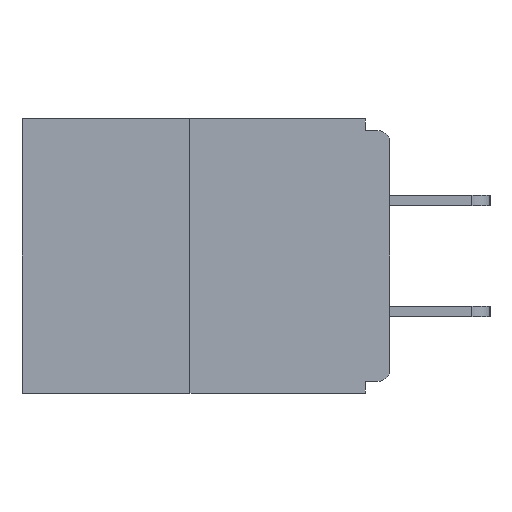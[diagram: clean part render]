
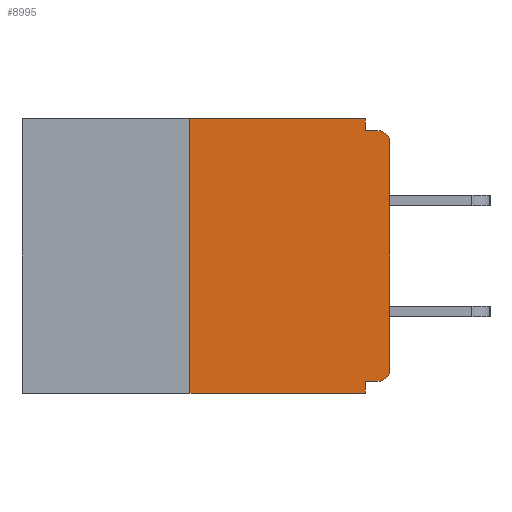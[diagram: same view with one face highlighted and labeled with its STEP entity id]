
A CAD part, left-side view. The second image highlights one B-rep face of the part: STEP entity #8995.
In plain terms, the highlighted planar face has unit normal (-1, 0, 0).
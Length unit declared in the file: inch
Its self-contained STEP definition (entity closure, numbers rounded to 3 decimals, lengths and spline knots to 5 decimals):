
#594 = VECTOR ( 'NONE', #9159, 39.37008 ) ;
#635 = CARTESIAN_POINT ( 'NONE',  ( 0., 0.25, 0. ) ) ;
#713 = EDGE_CURVE ( 'NONE', #4667, #17256, #10892, .T. ) ;
#949 = ORIENTED_EDGE ( 'NONE', *, *, #10261, .T. ) ;
#1646 = DIRECTION ( 'NONE',  ( 0., -1., 0. ) ) ;
#1842 = VERTEX_POINT ( 'NONE', #7702 ) ;
#2162 = CARTESIAN_POINT ( 'NONE',  ( 0., 0., -0.313 ) ) ;
#2696 = VECTOR ( 'NONE', #1646, 39.37008 ) ;
#2718 = LINE ( 'NONE', #14034, #6999 ) ;
#2818 = CARTESIAN_POINT ( 'NONE',  ( 0., 0.015, -0.328 ) ) ;
#2926 = VECTOR ( 'NONE', #5542, 39.37008 ) ;
#2937 = LINE ( 'NONE', #4559, #5231 ) ;
#3024 = DIRECTION ( 'NONE',  ( -1., 0., 0. ) ) ;
#3115 = VERTEX_POINT ( 'NONE', #3284 ) ;
#3284 = CARTESIAN_POINT ( 'NONE',  ( 0., 0.031, -0.343 ) ) ;
#3324 = AXIS2_PLACEMENT_3D ( 'NONE', #17347, #7849, #4935 ) ;
#3329 = CARTESIAN_POINT ( 'NONE',  ( 0., 0.015, -0.015 ) ) ;
#4559 = CARTESIAN_POINT ( 'NONE',  ( 0., 0.46, -0.343 ) ) ;
#4667 = VERTEX_POINT ( 'NONE', #2818 ) ;
#4835 = VERTEX_POINT ( 'NONE', #7347 ) ;
#4935 = DIRECTION ( 'NONE',  ( 0., 0., -1. ) ) ;
#5231 = VECTOR ( 'NONE', #15696, 39.37008 ) ;
#5542 = DIRECTION ( 'NONE',  ( 0., 0., -1. ) ) ;
#6225 = CARTESIAN_POINT ( 'NONE',  ( 0., 0.031, 0. ) ) ;
#6661 = DIRECTION ( 'NONE',  ( 0., 0., -1. ) ) ;
#6842 = VECTOR ( 'NONE', #16122, 39.37008 ) ;
#6853 = ORIENTED_EDGE ( 'NONE', *, *, #15094, .F. ) ;
#6999 = VECTOR ( 'NONE', #7064, 39.37008 ) ;
#7064 = DIRECTION ( 'NONE',  ( 0., 0., 1. ) ) ;
#7347 = CARTESIAN_POINT ( 'NONE',  ( 0., 0.031, -0.015 ) ) ;
#7702 = CARTESIAN_POINT ( 'NONE',  ( 0., 0.031, -0.328 ) ) ;
#7849 = DIRECTION ( 'NONE',  ( -1., 0., 0. ) ) ;
#8399 = VERTEX_POINT ( 'NONE', #6225 ) ;
#8420 = AXIS2_PLACEMENT_3D ( 'NONE', #14990, #16075, #6661 ) ;
#8628 = EDGE_LOOP ( 'NONE', ( #15716, #12999, #949, #6853, #9067, #8837, #11747, #15183, #16230, #17171 ) ) ;
#8713 = AXIS2_PLACEMENT_3D ( 'NONE', #12627, #3024, #10006 ) ;
#8716 = CARTESIAN_POINT ( 'NONE',  ( 0., 0., -0.015 ) ) ;
#8725 = VERTEX_POINT ( 'NONE', #11018 ) ;
#8774 = LINE ( 'NONE', #15549, #9151 ) ;
#8837 = ORIENTED_EDGE ( 'NONE', *, *, #713, .T. ) ;
#8982 = LINE ( 'NONE', #10603, #6842 ) ;
#8995 = ADVANCED_FACE ( 'NONE', ( #10563 ), #17625, .F. ) ;
#9004 = CIRCLE ( 'NONE', #8713, 0.015 ) ;
#9067 = ORIENTED_EDGE ( 'NONE', *, *, #15556, .F. ) ;
#9151 = VECTOR ( 'NONE', #15736, 39.37008 ) ;
#9159 = DIRECTION ( 'NONE',  ( 0., 0., 1. ) ) ;
#9624 = LINE ( 'NONE', #15143, #2926 ) ;
#9994 = CARTESIAN_POINT ( 'NONE',  ( 0., 0.25, -0.343 ) ) ;
#10006 = DIRECTION ( 'NONE',  ( 0., 0., -1. ) ) ;
#10261 = EDGE_CURVE ( 'NONE', #11356, #3115, #2937, .T. ) ;
#10321 = EDGE_CURVE ( 'NONE', #14365, #17772, #9004, .T. ) ;
#10563 = FACE_OUTER_BOUND ( 'NONE', #8628, .T. ) ;
#10603 = CARTESIAN_POINT ( 'NONE',  ( 0., 0., -0.328 ) ) ;
#10713 = EDGE_CURVE ( 'NONE', #8399, #4835, #9624, .T. ) ;
#10734 = EDGE_CURVE ( 'NONE', #4835, #17772, #16682, .T. ) ;
#10804 = CARTESIAN_POINT ( 'NONE',  ( 0., 0., -0.03 ) ) ;
#10892 = CIRCLE ( 'NONE', #3324, 0.015 ) ;
#10903 = EDGE_CURVE ( 'NONE', #11356, #8725, #15949, .T. ) ;
#11018 = CARTESIAN_POINT ( 'NONE',  ( 0., 0.25, 0. ) ) ;
#11079 = CARTESIAN_POINT ( 'NONE',  ( 0., 0.46, 0. ) ) ;
#11116 = EDGE_CURVE ( 'NONE', #17256, #14365, #2718, .T. ) ;
#11263 = LINE ( 'NONE', #11079, #2696 ) ;
#11356 = VERTEX_POINT ( 'NONE', #9994 ) ;
#11747 = ORIENTED_EDGE ( 'NONE', *, *, #11116, .T. ) ;
#12626 = EDGE_CURVE ( 'NONE', #8725, #8399, #11263, .T. ) ;
#12627 = CARTESIAN_POINT ( 'NONE',  ( 0., 0.015, -0.03 ) ) ;
#12999 = ORIENTED_EDGE ( 'NONE', *, *, #10903, .F. ) ;
#14034 = CARTESIAN_POINT ( 'NONE',  ( 0., 0., 0. ) ) ;
#14057 = DIRECTION ( 'NONE',  ( 0., -1., 0. ) ) ;
#14365 = VERTEX_POINT ( 'NONE', #10804 ) ;
#14990 = CARTESIAN_POINT ( 'NONE',  ( 0., 0.46, 0. ) ) ;
#15094 = EDGE_CURVE ( 'NONE', #1842, #3115, #8774, .T. ) ;
#15143 = CARTESIAN_POINT ( 'NONE',  ( 0., 0.031, 0. ) ) ;
#15183 = ORIENTED_EDGE ( 'NONE', *, *, #10321, .T. ) ;
#15549 = CARTESIAN_POINT ( 'NONE',  ( 0., 0.031, -0.343 ) ) ;
#15556 = EDGE_CURVE ( 'NONE', #4667, #1842, #8982, .T. ) ;
#15696 = DIRECTION ( 'NONE',  ( 0., -1., 0. ) ) ;
#15716 = ORIENTED_EDGE ( 'NONE', *, *, #12626, .F. ) ;
#15736 = DIRECTION ( 'NONE',  ( 0., 0., -1. ) ) ;
#15949 = LINE ( 'NONE', #635, #594 ) ;
#16075 = DIRECTION ( 'NONE',  ( 1., 0., 0. ) ) ;
#16122 = DIRECTION ( 'NONE',  ( 0., 1., 0. ) ) ;
#16230 = ORIENTED_EDGE ( 'NONE', *, *, #10734, .F. ) ;
#16682 = LINE ( 'NONE', #8716, #17105 ) ;
#17105 = VECTOR ( 'NONE', #14057, 39.37008 ) ;
#17171 = ORIENTED_EDGE ( 'NONE', *, *, #10713, .F. ) ;
#17256 = VERTEX_POINT ( 'NONE', #2162 ) ;
#17347 = CARTESIAN_POINT ( 'NONE',  ( 0., 0.015, -0.313 ) ) ;
#17625 = PLANE ( 'NONE',  #8420 ) ;
#17772 = VERTEX_POINT ( 'NONE', #3329 ) ;
